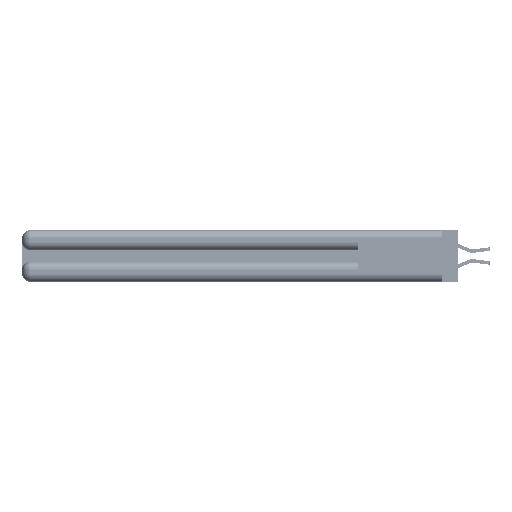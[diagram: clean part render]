
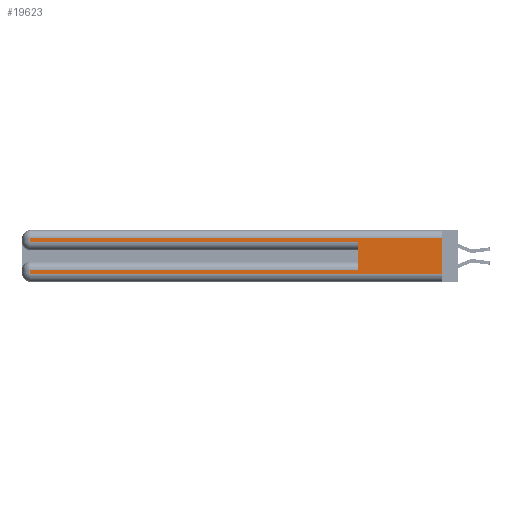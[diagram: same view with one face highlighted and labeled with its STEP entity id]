
A CAD part, left-side view. The second image highlights one B-rep face of the part: STEP entity #19623.
In plain terms, the highlighted planar face has unit normal (-1, 0, 0).
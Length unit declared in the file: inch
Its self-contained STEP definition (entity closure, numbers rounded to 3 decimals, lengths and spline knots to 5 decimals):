
#140 = CARTESIAN_POINT ( 'NONE',  ( 0., 0.6, 0.085 ) ) ;
#499 = CARTESIAN_POINT ( 'NONE',  ( 0., 0., 0.06 ) ) ;
#1567 = ORIENTED_EDGE ( 'NONE', *, *, #44000, .T. ) ;
#1996 = VECTOR ( 'NONE', #45506, 39.37008 ) ;
#2789 = VECTOR ( 'NONE', #30695, 39.37008 ) ;
#3917 = EDGE_CURVE ( 'NONE', #45181, #24678, #37333, .T. ) ;
#5815 = DIRECTION ( 'NONE',  ( 0., 0., 1. ) ) ;
#7739 = CARTESIAN_POINT ( 'NONE',  ( 0., 0., 0.37 ) ) ;
#7985 = CARTESIAN_POINT ( 'NONE',  ( 0., 0., 0.06 ) ) ;
#8623 = ORIENTED_EDGE ( 'NONE', *, *, #45033, .F. ) ;
#8735 = LINE ( 'NONE', #15774, #2789 ) ;
#8753 = VERTEX_POINT ( 'NONE', #140 ) ;
#11144 = EDGE_CURVE ( 'NONE', #38597, #26128, #24502, .T. ) ;
#11237 = LINE ( 'NONE', #36479, #30186 ) ;
#11385 = PLANE ( 'NONE',  #27054 ) ;
#12682 = DIRECTION ( 'NONE',  ( 0., 0., -1. ) ) ;
#13994 = DIRECTION ( 'NONE',  ( 0., -1., 0. ) ) ;
#14443 = ORIENTED_EDGE ( 'NONE', *, *, #11144, .T. ) ;
#14788 = ORIENTED_EDGE ( 'NONE', *, *, #47793, .T. ) ;
#14849 = VECTOR ( 'NONE', #34810, 39.37008 ) ;
#15497 = EDGE_CURVE ( 'NONE', #45181, #33087, #8735, .T. ) ;
#15774 = CARTESIAN_POINT ( 'NONE',  ( 0., 0., 0.37 ) ) ;
#16967 = CARTESIAN_POINT ( 'NONE',  ( 0., 2.94, 0.37 ) ) ;
#19623 = ADVANCED_FACE ( 'NONE', ( #43201 ), #11385, .F. ) ;
#20004 = EDGE_CURVE ( 'NONE', #36246, #27480, #11237, .T. ) ;
#20022 = ORIENTED_EDGE ( 'NONE', *, *, #40777, .T. ) ;
#20528 = LINE ( 'NONE', #40302, #38256 ) ;
#20915 = CARTESIAN_POINT ( 'NONE',  ( 0., 0.6, 0.285 ) ) ;
#21580 = CARTESIAN_POINT ( 'NONE',  ( 0., 2.94, 0.085 ) ) ;
#21604 = DIRECTION ( 'NONE',  ( 0., 1., 0. ) ) ;
#22493 = LINE ( 'NONE', #28618, #38502 ) ;
#22622 = CARTESIAN_POINT ( 'NONE',  ( 0., 2.94, 0.285 ) ) ;
#24178 = EDGE_LOOP ( 'NONE', ( #29470, #34875, #20022, #35457, #8623, #14788, #14443, #1567 ) ) ;
#24502 = LINE ( 'NONE', #44075, #29825 ) ;
#24678 = VERTEX_POINT ( 'NONE', #34065 ) ;
#26128 = VERTEX_POINT ( 'NONE', #46985 ) ;
#27054 = AXIS2_PLACEMENT_3D ( 'NONE', #7739, #30765, #34229 ) ;
#27480 = VERTEX_POINT ( 'NONE', #20915 ) ;
#28618 = CARTESIAN_POINT ( 'NONE',  ( 0., 0.6, 0.145 ) ) ;
#29470 = ORIENTED_EDGE ( 'NONE', *, *, #15497, .F. ) ;
#29825 = VECTOR ( 'NONE', #41107, 39.37008 ) ;
#30186 = VECTOR ( 'NONE', #13994, 39.37008 ) ;
#30695 = DIRECTION ( 'NONE',  ( 0., 0., -1. ) ) ;
#30765 = DIRECTION ( 'NONE',  ( 1., 0., 0. ) ) ;
#32874 = VECTOR ( 'NONE', #12682, 39.37008 ) ;
#33087 = VERTEX_POINT ( 'NONE', #499 ) ;
#33363 = LINE ( 'NONE', #7985, #1996 ) ;
#34065 = CARTESIAN_POINT ( 'NONE',  ( 0., 2.94, 0.31 ) ) ;
#34229 = DIRECTION ( 'NONE',  ( 0., 0., -1. ) ) ;
#34810 = DIRECTION ( 'NONE',  ( 0., 1., 0. ) ) ;
#34875 = ORIENTED_EDGE ( 'NONE', *, *, #3917, .T. ) ;
#34965 = CARTESIAN_POINT ( 'NONE',  ( 0., 0., 0.31 ) ) ;
#35457 = ORIENTED_EDGE ( 'NONE', *, *, #20004, .T. ) ;
#36246 = VERTEX_POINT ( 'NONE', #22622 ) ;
#36479 = CARTESIAN_POINT ( 'NONE',  ( 0., 0., 0.285 ) ) ;
#37333 = LINE ( 'NONE', #34965, #14849 ) ;
#38256 = VECTOR ( 'NONE', #21604, 39.37008 ) ;
#38502 = VECTOR ( 'NONE', #5815, 39.37008 ) ;
#38597 = VERTEX_POINT ( 'NONE', #21580 ) ;
#40302 = CARTESIAN_POINT ( 'NONE',  ( 0., 0., 0.085 ) ) ;
#40777 = EDGE_CURVE ( 'NONE', #24678, #36246, #44065, .T. ) ;
#41107 = DIRECTION ( 'NONE',  ( 0., 0., -1. ) ) ;
#43201 = FACE_OUTER_BOUND ( 'NONE', #24178, .T. ) ;
#43952 = CARTESIAN_POINT ( 'NONE',  ( 0., 0., 0.31 ) ) ;
#44000 = EDGE_CURVE ( 'NONE', #26128, #33087, #33363, .T. ) ;
#44065 = LINE ( 'NONE', #16967, #32874 ) ;
#44075 = CARTESIAN_POINT ( 'NONE',  ( 0., 2.94, 0.37 ) ) ;
#45033 = EDGE_CURVE ( 'NONE', #8753, #27480, #22493, .T. ) ;
#45181 = VERTEX_POINT ( 'NONE', #43952 ) ;
#45506 = DIRECTION ( 'NONE',  ( 0., -1., 0. ) ) ;
#46985 = CARTESIAN_POINT ( 'NONE',  ( 0., 2.94, 0.06 ) ) ;
#47793 = EDGE_CURVE ( 'NONE', #8753, #38597, #20528, .T. ) ;
